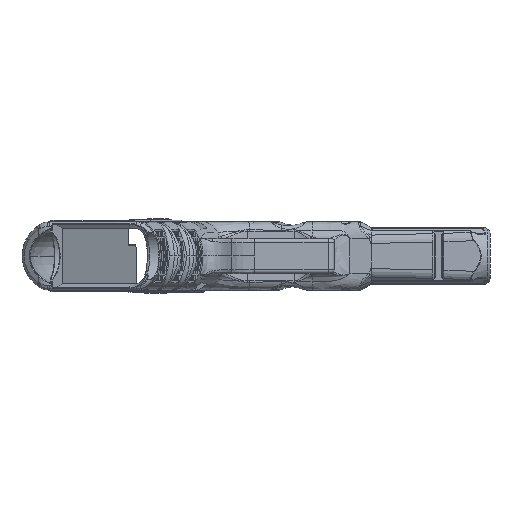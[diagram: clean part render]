
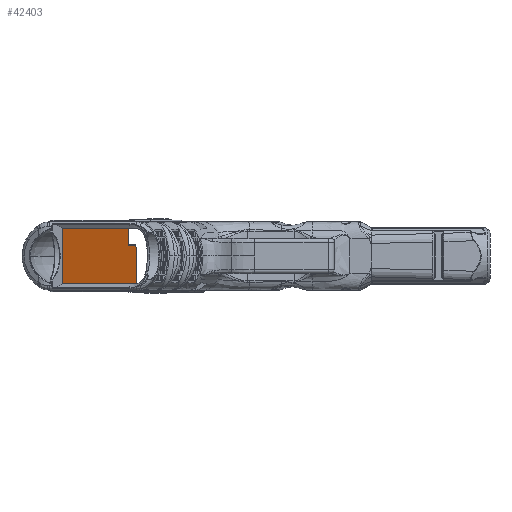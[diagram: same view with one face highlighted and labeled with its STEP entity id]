
A CAD part, front view. The second image highlights one B-rep face of the part: STEP entity #42403.
In plain terms, the highlighted planar face has unit normal (0.951, -0.309, 0).
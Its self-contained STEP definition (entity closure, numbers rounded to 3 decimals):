
#1782=LINE('',#69803,#4510);
#1783=LINE('',#69847,#4511);
#1784=LINE('',#69850,#4512);
#1785=LINE('',#69852,#4513);
#1786=LINE('',#69854,#4514);
#1787=LINE('',#69855,#4515);
#4510=VECTOR('',#49829,10.);
#4511=VECTOR('',#49840,10.);
#4512=VECTOR('',#49843,10.);
#4513=VECTOR('',#49844,1000.);
#4514=VECTOR('',#49845,10.);
#4515=VECTOR('',#49846,1000.);
#6915=PLANE('',#45137);
#7858=ELLIPSE('',#45134,0.536,0.51);
#9361=FACE_OUTER_BOUND('',#11898,.T.);
#11898=EDGE_LOOP('',(#29233,#29234,#29235,#29236,#29237,#29238,#29239));
#17375=VERTEX_POINT('',#69800);
#17376=VERTEX_POINT('',#69802);
#17377=VERTEX_POINT('',#69841);
#17378=VERTEX_POINT('',#69845);
#17379=VERTEX_POINT('',#69849);
#17380=VERTEX_POINT('',#69851);
#17381=VERTEX_POINT('',#69853);
#21937=EDGE_CURVE('',#17375,#17376,#1782,.T.);
#21940=EDGE_CURVE('',#17377,#17375,#7858,.T.);
#21942=EDGE_CURVE('',#17378,#17377,#1783,.T.);
#21943=EDGE_CURVE('',#17379,#17378,#1784,.T.);
#21944=EDGE_CURVE('',#17380,#17379,#1785,.T.);
#21945=EDGE_CURVE('',#17381,#17380,#1786,.T.);
#21946=EDGE_CURVE('',#17376,#17381,#1787,.T.);
#29233=ORIENTED_EDGE('',*,*,#21943,.F.);
#29234=ORIENTED_EDGE('',*,*,#21944,.F.);
#29235=ORIENTED_EDGE('',*,*,#21945,.F.);
#29236=ORIENTED_EDGE('',*,*,#21946,.F.);
#29237=ORIENTED_EDGE('',*,*,#21937,.F.);
#29238=ORIENTED_EDGE('',*,*,#21940,.F.);
#29239=ORIENTED_EDGE('',*,*,#21942,.F.);
#42403=ADVANCED_FACE('',(#9361),#6915,.F.);
#45134=AXIS2_PLACEMENT_3D('',#69843,#49834,#49835);
#45137=AXIS2_PLACEMENT_3D('',#69848,#49841,#49842);
#49829=DIRECTION('',(0.,0.,-1.));
#49834=DIRECTION('center_axis',(-0.951,0.309,0.));
#49835=DIRECTION('ref_axis',(0.309,0.951,0.));
#49840=DIRECTION('',(0.309,0.951,0.));
#49841=DIRECTION('center_axis',(-0.951,0.309,0.));
#49842=DIRECTION('ref_axis',(0.,0.,1.));
#49843=DIRECTION('',(0.,0.,-1.));
#49844=DIRECTION('',(0.309,0.951,0.));
#49845=DIRECTION('',(0.,0.,1.));
#49846=DIRECTION('',(-0.309,-0.951,0.));
#69800=CARTESIAN_POINT('',(33.382,-2.141,3.75));
#69802=CARTESIAN_POINT('',(33.382,-2.141,-11.75));
#69803=CARTESIAN_POINT('',(33.382,-2.141,-5.651));
#69841=CARTESIAN_POINT('',(33.216,-2.651,4.26));
#69843=CARTESIAN_POINT('Origin',(33.216,-2.651,3.75));
#69845=CARTESIAN_POINT('',(30.049,-12.4,4.26));
#69847=CARTESIAN_POINT('',(34.619,1.664,4.26));
#69848=CARTESIAN_POINT('Origin',(33.829,-0.765,-11.75));
#69849=CARTESIAN_POINT('',(30.049,-12.4,11.75));
#69850=CARTESIAN_POINT('',(30.049,-12.4,2.982));
#69851=CARTESIAN_POINT('',(2.236,-98.,11.75));
#69852=CARTESIAN_POINT('',(30.125,-12.165,11.75));
#69853=CARTESIAN_POINT('',(2.236,-98.,-11.75));
#69854=CARTESIAN_POINT('',(2.236,-98.,-18.375));
#69855=CARTESIAN_POINT('',(33.829,-0.765,-11.75));
